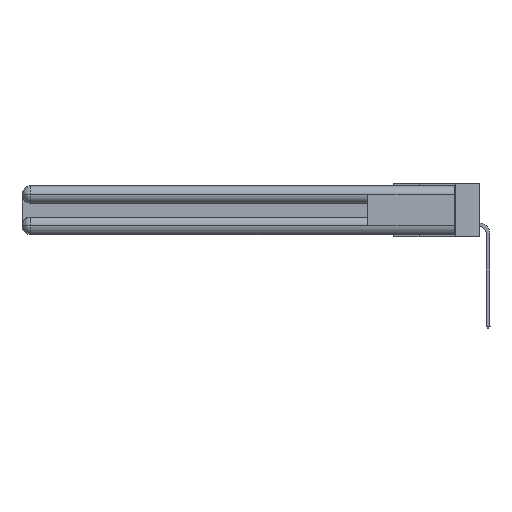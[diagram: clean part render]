
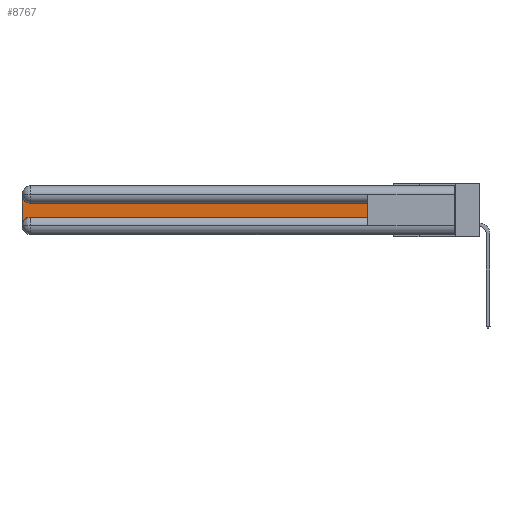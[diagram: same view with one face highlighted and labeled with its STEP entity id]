
A CAD part, left-side view. The second image highlights one B-rep face of the part: STEP entity #8767.
In plain terms, the highlighted planar face has unit normal (-1, 0, 0).
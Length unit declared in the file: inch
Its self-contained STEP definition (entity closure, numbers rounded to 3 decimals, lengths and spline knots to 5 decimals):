
#1038 = CARTESIAN_POINT ( 'NONE',  ( 0.075, 0.6, -0.1225 ) ) ;
#2012 = ORIENTED_EDGE ( 'NONE', *, *, #13812, .T. ) ;
#3001 = VECTOR ( 'NONE', #20971, 39.37008 ) ;
#3587 = EDGE_CURVE ( 'NONE', #14331, #27093, #28349, .T. ) ;
#3698 = CARTESIAN_POINT ( 'NONE',  ( 0.075, 3., -0.0625 ) ) ;
#3751 = ORIENTED_EDGE ( 'NONE', *, *, #17459, .T. ) ;
#3823 = CIRCLE ( 'NONE', #19458, 0.06 ) ;
#3965 = CARTESIAN_POINT ( 'NONE',  ( 0.075, 2.94, -0.0625 ) ) ;
#4016 = DIRECTION ( 'NONE',  ( 1., 0., 0. ) ) ;
#4125 = CARTESIAN_POINT ( 'NONE',  ( 0.075, 3., -0.1225 ) ) ;
#5094 = DIRECTION ( 'NONE',  ( 0., 0., 1. ) ) ;
#5116 = LINE ( 'NONE', #26115, #22394 ) ;
#5456 = CARTESIAN_POINT ( 'NONE',  ( 0.075, 2.94, -0.1225 ) ) ;
#6217 = VECTOR ( 'NONE', #25981, 39.37008 ) ;
#6363 = LINE ( 'NONE', #24266, #28322 ) ;
#6452 = EDGE_CURVE ( 'NONE', #22836, #14593, #19404, .T. ) ;
#8712 = ORIENTED_EDGE ( 'NONE', *, *, #18465, .T. ) ;
#8767 = ADVANCED_FACE ( 'NONE', ( #28024 ), #29530, .F. ) ;
#9229 = ORIENTED_EDGE ( 'NONE', *, *, #3587, .T. ) ;
#9266 = LINE ( 'NONE', #23531, #3001 ) ;
#9933 = DIRECTION ( 'NONE',  ( 1., 0., 0. ) ) ;
#12177 = DIRECTION ( 'NONE',  ( 0., 0., -1. ) ) ;
#13812 = EDGE_CURVE ( 'NONE', #20006, #22836, #3823, .T. ) ;
#14331 = VERTEX_POINT ( 'NONE', #5456 ) ;
#14573 = CARTESIAN_POINT ( 'NONE',  ( 0.075, 2.94, -0.2775 ) ) ;
#14593 = VERTEX_POINT ( 'NONE', #25279 ) ;
#14641 = CARTESIAN_POINT ( 'NONE',  ( 0.075, 3., -0.2775 ) ) ;
#17459 = EDGE_CURVE ( 'NONE', #19004, #14331, #9266, .T. ) ;
#18032 = DIRECTION ( 'NONE',  ( 1., 0., 0. ) ) ;
#18465 = EDGE_CURVE ( 'NONE', #14593, #19004, #5116, .T. ) ;
#19004 = VERTEX_POINT ( 'NONE', #1038 ) ;
#19258 = DIRECTION ( 'NONE',  ( 0., 0., -1. ) ) ;
#19404 = LINE ( 'NONE', #28432, #6217 ) ;
#19458 = AXIS2_PLACEMENT_3D ( 'NONE', #14573, #9933, #19258 ) ;
#19962 = DIRECTION ( 'NONE',  ( 0., 0., -1. ) ) ;
#19975 = EDGE_CURVE ( 'NONE', #27093, #20006, #6363, .T. ) ;
#20006 = VERTEX_POINT ( 'NONE', #14641 ) ;
#20971 = DIRECTION ( 'NONE',  ( 0., 1., 0. ) ) ;
#21503 = ORIENTED_EDGE ( 'NONE', *, *, #19975, .T. ) ;
#22394 = VECTOR ( 'NONE', #5094, 39.37008 ) ;
#22499 = ORIENTED_EDGE ( 'NONE', *, *, #6452, .T. ) ;
#22787 = DIRECTION ( 'NONE',  ( 0., 0., -1. ) ) ;
#22836 = VERTEX_POINT ( 'NONE', #26326 ) ;
#23531 = CARTESIAN_POINT ( 'NONE',  ( 0.075, 0.6, -0.1225 ) ) ;
#24266 = CARTESIAN_POINT ( 'NONE',  ( 0.075, 3., -0.2175 ) ) ;
#25279 = CARTESIAN_POINT ( 'NONE',  ( 0.075, 0.6, -0.2175 ) ) ;
#25981 = DIRECTION ( 'NONE',  ( 0., -1., 0. ) ) ;
#26115 = CARTESIAN_POINT ( 'NONE',  ( 0.075, 0.6, -0.2175 ) ) ;
#26326 = CARTESIAN_POINT ( 'NONE',  ( 0.075, 2.94, -0.2175 ) ) ;
#27093 = VERTEX_POINT ( 'NONE', #3698 ) ;
#27388 = AXIS2_PLACEMENT_3D ( 'NONE', #3965, #18032, #19962 ) ;
#27639 = AXIS2_PLACEMENT_3D ( 'NONE', #4125, #4016, #22787 ) ;
#28024 = FACE_OUTER_BOUND ( 'NONE', #29174, .T. ) ;
#28322 = VECTOR ( 'NONE', #12177, 39.37008 ) ;
#28349 = CIRCLE ( 'NONE', #27388, 0.06 ) ;
#28432 = CARTESIAN_POINT ( 'NONE',  ( 0.075, 0.6, -0.2175 ) ) ;
#29174 = EDGE_LOOP ( 'NONE', ( #3751, #9229, #21503, #2012, #22499, #8712 ) ) ;
#29530 = PLANE ( 'NONE',  #27639 ) ;
